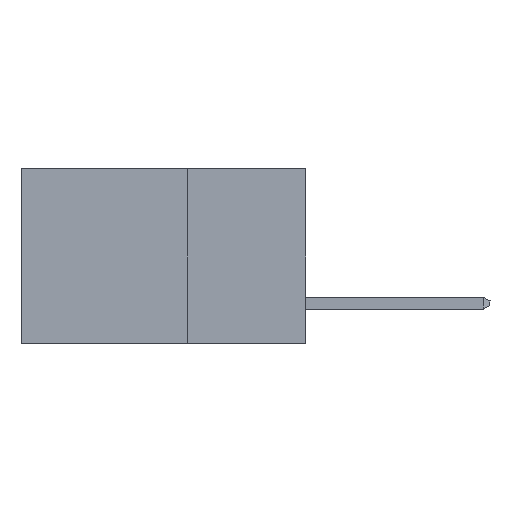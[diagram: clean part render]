
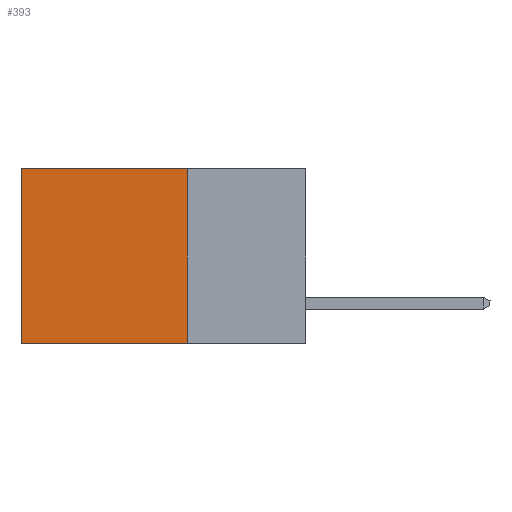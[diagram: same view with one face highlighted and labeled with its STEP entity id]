
A CAD part, left-side view. The second image highlights one B-rep face of the part: STEP entity #393.
In plain terms, the highlighted planar face has unit normal (-1, 0, 0).
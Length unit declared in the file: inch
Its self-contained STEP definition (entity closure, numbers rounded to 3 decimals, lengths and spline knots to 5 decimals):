
#38 = CARTESIAN_POINT ( 'NONE',  ( 0.2615, 0.6, 0. ) ) ;
#242 = LINE ( 'NONE', #10343, #3939 ) ;
#393 = ADVANCED_FACE ( 'NONE', ( #3255 ), #6086, .F. ) ;
#632 = LINE ( 'NONE', #9586, #8550 ) ;
#1250 = VECTOR ( 'NONE', #8323, 39.37008 ) ;
#1529 = VERTEX_POINT ( 'NONE', #7364 ) ;
#1603 = VERTEX_POINT ( 'NONE', #7668 ) ;
#1951 = ORIENTED_EDGE ( 'NONE', *, *, #4378, .F. ) ;
#2213 = DIRECTION ( 'NONE',  ( 0., 0., -1. ) ) ;
#2329 = DIRECTION ( 'NONE',  ( 0., 0., -1. ) ) ;
#2883 = ORIENTED_EDGE ( 'NONE', *, *, #6321, .T. ) ;
#2947 = VERTEX_POINT ( 'NONE', #9729 ) ;
#3240 = LINE ( 'NONE', #3480, #4917 ) ;
#3255 = FACE_OUTER_BOUND ( 'NONE', #9216, .T. ) ;
#3480 = CARTESIAN_POINT ( 'NONE',  ( 0.2615, 0.6, -0.37 ) ) ;
#3939 = VECTOR ( 'NONE', #10506, 39.37008 ) ;
#4378 = EDGE_CURVE ( 'NONE', #1603, #1529, #632, .T. ) ;
#4438 = AXIS2_PLACEMENT_3D ( 'NONE', #10621, #5005, #4895 ) ;
#4706 = LINE ( 'NONE', #10207, #1250 ) ;
#4895 = DIRECTION ( 'NONE',  ( 0., 0., -1. ) ) ;
#4917 = VECTOR ( 'NONE', #2329, 39.37008 ) ;
#5005 = DIRECTION ( 'NONE',  ( 1., 0., 0. ) ) ;
#5934 = EDGE_CURVE ( 'NONE', #1529, #2947, #4706, .T. ) ;
#6086 = PLANE ( 'NONE',  #4438 ) ;
#6321 = EDGE_CURVE ( 'NONE', #10713, #2947, #3240, .T. ) ;
#7364 = CARTESIAN_POINT ( 'NONE',  ( 0.2615, 0.25, -0.37 ) ) ;
#7668 = CARTESIAN_POINT ( 'NONE',  ( 0.2615, 0.25, 0. ) ) ;
#8323 = DIRECTION ( 'NONE',  ( 0., 1., 0. ) ) ;
#8550 = VECTOR ( 'NONE', #2213, 39.37008 ) ;
#9216 = EDGE_LOOP ( 'NONE', ( #2883, #9260, #1951, #11711 ) ) ;
#9260 = ORIENTED_EDGE ( 'NONE', *, *, #5934, .F. ) ;
#9586 = CARTESIAN_POINT ( 'NONE',  ( 0.2615, 0.25, -0.37 ) ) ;
#9729 = CARTESIAN_POINT ( 'NONE',  ( 0.2615, 0.6, -0.37 ) ) ;
#10207 = CARTESIAN_POINT ( 'NONE',  ( 0.2615, 0.25, -0.37 ) ) ;
#10343 = CARTESIAN_POINT ( 'NONE',  ( 0.2615, 0.25, 0. ) ) ;
#10506 = DIRECTION ( 'NONE',  ( 0., 1., 0. ) ) ;
#10621 = CARTESIAN_POINT ( 'NONE',  ( 0.2615, 0.25, -0.37 ) ) ;
#10713 = VERTEX_POINT ( 'NONE', #38 ) ;
#11711 = ORIENTED_EDGE ( 'NONE', *, *, #11762, .T. ) ;
#11762 = EDGE_CURVE ( 'NONE', #1603, #10713, #242, .T. ) ;
